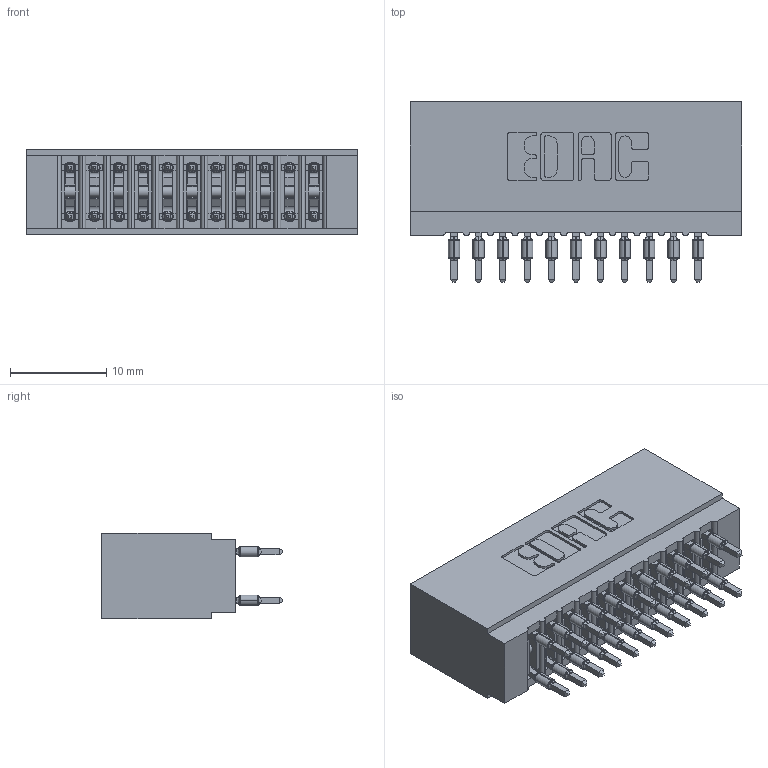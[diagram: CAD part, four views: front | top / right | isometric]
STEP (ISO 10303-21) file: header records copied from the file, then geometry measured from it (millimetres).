
FILE_DESCRIPTION (( 'STEP AP203' ), '1' );
FILE_NAME ('725-022-560-201.STEP', '2026-02-24T16:55:56', ( '' ), ( '' ), 'SwSTEP 2.0', 'SolidWorks 2023', '' );
FILE_SCHEMA (( 'CONFIG_CONTROL_DESIGN' ));
Length unit declared in the file: millimetre
Products named in the file (3): 725-022-560-201; 725 Part_Insulator Option - 01; 745-292-001_560
Assembly tree (23 placements, depth 2):
  725-022-560-201
    725 Part_Insulator Option - 01
    745-292-001_560  x22
Bounding box: 34.54 x 18.8 x 8.89 mm (x, y, z)
Volume: 2976.8 mm3; surface area: 5971.3 mm2
Topology: 23 solids, 23 shells, 2262 faces, 6183 edges, 3930 vertices
Faces by surface type: plane 1177, cylinder 513, bspline 440, torus 132
Entity records: 23038 total; most frequent: CARTESIAN_POINT 4509, ORIENTED_EDGE 3882, DIRECTION 3425, EDGE_CURVE 1941, LINE 1685, VECTOR 1685, VERTEX_POINT 1242, AXIS2_PLACEMENT_3D 870
